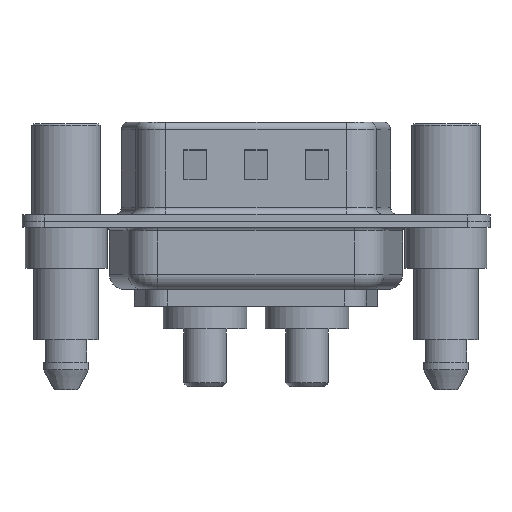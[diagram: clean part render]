
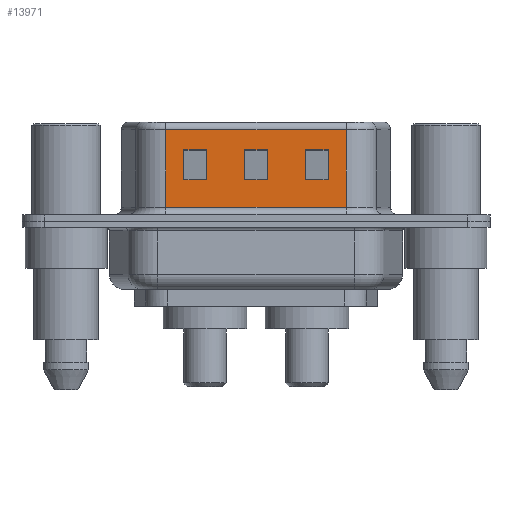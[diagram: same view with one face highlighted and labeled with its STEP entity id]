
A CAD part, front view. The second image highlights one B-rep face of the part: STEP entity #13971.
In plain terms, the highlighted planar face has unit normal (0, -1, 0).
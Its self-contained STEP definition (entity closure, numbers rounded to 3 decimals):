
#172 = ORIENTED_EDGE ( 'NONE', *, *, #3386, .T. ) ;
#312 = PLANE ( 'NONE',  #12721 ) ;
#315 = VECTOR ( 'NONE', #2605, 1000. ) ;
#353 = EDGE_CURVE ( 'NONE', #12784, #11285, #8005, .T. ) ;
#548 = ORIENTED_EDGE ( 'NONE', *, *, #11275, .T. ) ;
#585 = EDGE_LOOP ( 'NONE', ( #6959, #7529, #548, #10869 ) ) ;
#978 = FACE_BOUND ( 'NONE', #1813, .T. ) ;
#1166 = CARTESIAN_POINT ( 'NONE',  ( 22.45, -4.58, 2.705 ) ) ;
#1173 = LINE ( 'NONE', #1695, #9858 ) ;
#1420 = CARTESIAN_POINT ( 'NONE',  ( 18.45, -4.58, 6.52 ) ) ;
#1442 = CARTESIAN_POINT ( 'NONE',  ( 9.25, -4.58, 2.705 ) ) ;
#1467 = DIRECTION ( 'NONE',  ( 0., 1., 0. ) ) ;
#1602 = VERTEX_POINT ( 'NONE', #9291 ) ;
#1667 = CARTESIAN_POINT ( 'NONE',  ( 13.25, -4.58, 6.52 ) ) ;
#1695 = CARTESIAN_POINT ( 'NONE',  ( 18.45, -4.58, 0.9 ) ) ;
#1702 = VECTOR ( 'NONE', #13607, 1000. ) ;
#1726 = VECTOR ( 'NONE', #2439, 1000. ) ;
#1745 = CARTESIAN_POINT ( 'NONE',  ( 18.45, -4.58, 2.705 ) ) ;
#1813 = EDGE_LOOP ( 'NONE', ( #6625, #8859, #172, #13613 ) ) ;
#1853 = EDGE_CURVE ( 'NONE', #9168, #2019, #5000, .T. ) ;
#1959 = VECTOR ( 'NONE', #5001, 1000. ) ;
#2019 = VERTEX_POINT ( 'NONE', #8763 ) ;
#2021 = VECTOR ( 'NONE', #11871, 1000. ) ;
#2028 = FACE_OUTER_BOUND ( 'NONE', #12040, .T. ) ;
#2131 = EDGE_CURVE ( 'NONE', #2898, #1602, #7871, .T. ) ;
#2439 = DIRECTION ( 'NONE',  ( 0., 0., -1. ) ) ;
#2518 = CARTESIAN_POINT ( 'NONE',  ( 15.75, -4.58, 2.705 ) ) ;
#2572 = ORIENTED_EDGE ( 'NONE', *, *, #7505, .T. ) ;
#2605 = DIRECTION ( 'NONE',  ( -1., 0., 0. ) ) ;
#2628 = EDGE_CURVE ( 'NONE', #9487, #6154, #5510, .T. ) ;
#2898 = VERTEX_POINT ( 'NONE', #4306 ) ;
#3002 = CARTESIAN_POINT ( 'NONE',  ( 6.55, -4.58, 6.02 ) ) ;
#3151 = VECTOR ( 'NONE', #10732, 1000. ) ;
#3168 = VERTEX_POINT ( 'NONE', #2518 ) ;
#3368 = CARTESIAN_POINT ( 'NONE',  ( 17.25, -4.58, 6.52 ) ) ;
#3386 = EDGE_CURVE ( 'NONE', #13891, #9487, #7127, .T. ) ;
#3643 = ORIENTED_EDGE ( 'NONE', *, *, #5201, .T. ) ;
#3783 = DIRECTION ( 'NONE',  ( -1., 0., 0. ) ) ;
#3884 = EDGE_CURVE ( 'NONE', #11285, #6848, #10783, .T. ) ;
#4009 = DIRECTION ( 'NONE',  ( -1., 0., 0. ) ) ;
#4306 = CARTESIAN_POINT ( 'NONE',  ( 13.25, -4.58, 2.705 ) ) ;
#4501 = CARTESIAN_POINT ( 'NONE',  ( 18.45, -4.58, 6.52 ) ) ;
#4917 = EDGE_CURVE ( 'NONE', #11046, #13891, #9039, .T. ) ;
#5000 = LINE ( 'NONE', #3368, #1959 ) ;
#5001 = DIRECTION ( 'NONE',  ( 0., 0., -1. ) ) ;
#5065 = LINE ( 'NONE', #10719, #2021 ) ;
#5129 = VECTOR ( 'NONE', #6635, 1000. ) ;
#5201 = EDGE_CURVE ( 'NONE', #9358, #2898, #6180, .T. ) ;
#5401 = VERTEX_POINT ( 'NONE', #13269 ) ;
#5510 = LINE ( 'NONE', #12932, #8553 ) ;
#5630 = DIRECTION ( 'NONE',  ( 0., 0., -1. ) ) ;
#5995 = DIRECTION ( 'NONE',  ( 1., 0., 0. ) ) ;
#6060 = EDGE_CURVE ( 'NONE', #12784, #14525, #11647, .T. ) ;
#6154 = VERTEX_POINT ( 'NONE', #9164 ) ;
#6180 = LINE ( 'NONE', #1667, #3151 ) ;
#6207 = VECTOR ( 'NONE', #5995, 1000. ) ;
#6216 = DIRECTION ( 'NONE',  ( 1., 0., 0. ) ) ;
#6446 = CARTESIAN_POINT ( 'NONE',  ( 11.75, -4.58, 4.705 ) ) ;
#6625 = ORIENTED_EDGE ( 'NONE', *, *, #10972, .T. ) ;
#6635 = DIRECTION ( 'NONE',  ( 0., 0., -1. ) ) ;
#6848 = VERTEX_POINT ( 'NONE', #7420 ) ;
#6959 = ORIENTED_EDGE ( 'NONE', *, *, #1853, .T. ) ;
#7127 = LINE ( 'NONE', #12329, #12730 ) ;
#7420 = CARTESIAN_POINT ( 'NONE',  ( 6.55, -4.58, 0.9 ) ) ;
#7505 = EDGE_CURVE ( 'NONE', #11313, #9358, #5065, .T. ) ;
#7529 = ORIENTED_EDGE ( 'NONE', *, *, #12021, .T. ) ;
#7566 = CARTESIAN_POINT ( 'NONE',  ( 15.75, -4.58, 6.52 ) ) ;
#7620 = DIRECTION ( 'NONE',  ( 0., 0., 1. ) ) ;
#7871 = LINE ( 'NONE', #1745, #10494 ) ;
#8005 = LINE ( 'NONE', #13865, #13585 ) ;
#8553 = VECTOR ( 'NONE', #12454, 1000. ) ;
#8763 = CARTESIAN_POINT ( 'NONE',  ( 17.25, -4.58, 2.705 ) ) ;
#8859 = ORIENTED_EDGE ( 'NONE', *, *, #4917, .T. ) ;
#9039 = LINE ( 'NONE', #9404, #315 ) ;
#9164 = CARTESIAN_POINT ( 'NONE',  ( 9.25, -4.58, 4.705 ) ) ;
#9168 = VERTEX_POINT ( 'NONE', #11409 ) ;
#9219 = CARTESIAN_POINT ( 'NONE',  ( 7.75, -4.58, 2.705 ) ) ;
#9241 = LINE ( 'NONE', #10509, #6207 ) ;
#9291 = CARTESIAN_POINT ( 'NONE',  ( 11.75, -4.58, 2.705 ) ) ;
#9358 = VERTEX_POINT ( 'NONE', #11985 ) ;
#9404 = CARTESIAN_POINT ( 'NONE',  ( 14.45, -4.58, 2.705 ) ) ;
#9407 = DIRECTION ( 'NONE',  ( 0., 0., 1. ) ) ;
#9487 = VERTEX_POINT ( 'NONE', #12237 ) ;
#9750 = EDGE_CURVE ( 'NONE', #5401, #9168, #9241, .T. ) ;
#9858 = VECTOR ( 'NONE', #6216, 1000. ) ;
#9890 = VECTOR ( 'NONE', #10934, 1000. ) ;
#10397 = FACE_BOUND ( 'NONE', #585, .T. ) ;
#10431 = CARTESIAN_POINT ( 'NONE',  ( 9.25, -4.58, 6.52 ) ) ;
#10494 = VECTOR ( 'NONE', #4009, 1000. ) ;
#10509 = CARTESIAN_POINT ( 'NONE',  ( 22.45, -4.58, 4.705 ) ) ;
#10662 = ORIENTED_EDGE ( 'NONE', *, *, #2131, .T. ) ;
#10719 = CARTESIAN_POINT ( 'NONE',  ( 18.45, -4.58, 4.705 ) ) ;
#10720 = VECTOR ( 'NONE', #7620, 1000. ) ;
#10732 = DIRECTION ( 'NONE',  ( 0., 0., -1. ) ) ;
#10747 = LINE ( 'NONE', #1166, #1702 ) ;
#10783 = LINE ( 'NONE', #14458, #5129 ) ;
#10869 = ORIENTED_EDGE ( 'NONE', *, *, #9750, .T. ) ;
#10934 = DIRECTION ( 'NONE',  ( 0., 0., 1. ) ) ;
#10972 = EDGE_CURVE ( 'NONE', #6154, #11046, #13407, .T. ) ;
#11032 = ORIENTED_EDGE ( 'NONE', *, *, #353, .T. ) ;
#11046 = VERTEX_POINT ( 'NONE', #1442 ) ;
#11275 = EDGE_CURVE ( 'NONE', #3168, #5401, #14248, .T. ) ;
#11285 = VERTEX_POINT ( 'NONE', #3002 ) ;
#11298 = EDGE_LOOP ( 'NONE', ( #2572, #3643, #10662, #14244 ) ) ;
#11313 = VERTEX_POINT ( 'NONE', #6446 ) ;
#11409 = CARTESIAN_POINT ( 'NONE',  ( 17.25, -4.58, 4.705 ) ) ;
#11452 = LINE ( 'NONE', #13186, #10720 ) ;
#11644 = CARTESIAN_POINT ( 'NONE',  ( 18.45, -4.58, 6.02 ) ) ;
#11647 = LINE ( 'NONE', #4501, #14236 ) ;
#11871 = DIRECTION ( 'NONE',  ( 1., 0., 0. ) ) ;
#11985 = CARTESIAN_POINT ( 'NONE',  ( 13.25, -4.58, 4.705 ) ) ;
#12021 = EDGE_CURVE ( 'NONE', #2019, #3168, #10747, .T. ) ;
#12040 = EDGE_LOOP ( 'NONE', ( #12510, #11032, #13755, #13781 ) ) ;
#12237 = CARTESIAN_POINT ( 'NONE',  ( 7.75, -4.58, 4.705 ) ) ;
#12316 = EDGE_CURVE ( 'NONE', #6848, #14525, #1173, .T. ) ;
#12329 = CARTESIAN_POINT ( 'NONE',  ( 7.75, -4.58, 6.52 ) ) ;
#12454 = DIRECTION ( 'NONE',  ( 1., 0., 0. ) ) ;
#12510 = ORIENTED_EDGE ( 'NONE', *, *, #6060, .F. ) ;
#12578 = CARTESIAN_POINT ( 'NONE',  ( 18.45, -4.58, 0.9 ) ) ;
#12721 = AXIS2_PLACEMENT_3D ( 'NONE', #1420, #1467, #9407 ) ;
#12730 = VECTOR ( 'NONE', #14467, 1000. ) ;
#12784 = VERTEX_POINT ( 'NONE', #11644 ) ;
#12932 = CARTESIAN_POINT ( 'NONE',  ( 14.45, -4.58, 4.705 ) ) ;
#13026 = EDGE_CURVE ( 'NONE', #1602, #11313, #11452, .T. ) ;
#13186 = CARTESIAN_POINT ( 'NONE',  ( 11.75, -4.58, 6.52 ) ) ;
#13269 = CARTESIAN_POINT ( 'NONE',  ( 15.75, -4.58, 4.705 ) ) ;
#13348 = FACE_BOUND ( 'NONE', #11298, .T. ) ;
#13407 = LINE ( 'NONE', #10431, #1726 ) ;
#13585 = VECTOR ( 'NONE', #3783, 1000. ) ;
#13607 = DIRECTION ( 'NONE',  ( -1., 0., 0. ) ) ;
#13613 = ORIENTED_EDGE ( 'NONE', *, *, #2628, .T. ) ;
#13755 = ORIENTED_EDGE ( 'NONE', *, *, #3884, .T. ) ;
#13781 = ORIENTED_EDGE ( 'NONE', *, *, #12316, .T. ) ;
#13865 = CARTESIAN_POINT ( 'NONE',  ( 18.45, -4.58, 6.02 ) ) ;
#13891 = VERTEX_POINT ( 'NONE', #9219 ) ;
#13971 = ADVANCED_FACE ( 'NONE', ( #978, #10397, #13348, #2028 ), #312, .F. ) ;
#14236 = VECTOR ( 'NONE', #5630, 1000. ) ;
#14244 = ORIENTED_EDGE ( 'NONE', *, *, #13026, .T. ) ;
#14248 = LINE ( 'NONE', #7566, #9890 ) ;
#14458 = CARTESIAN_POINT ( 'NONE',  ( 6.55, -4.58, 6.52 ) ) ;
#14467 = DIRECTION ( 'NONE',  ( 0., 0., 1. ) ) ;
#14525 = VERTEX_POINT ( 'NONE', #12578 ) ;
